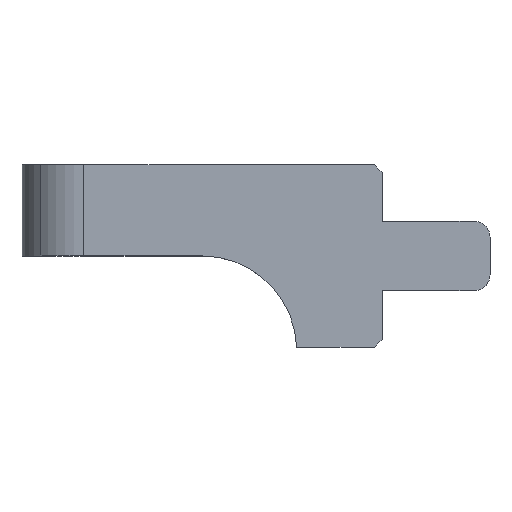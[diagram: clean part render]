
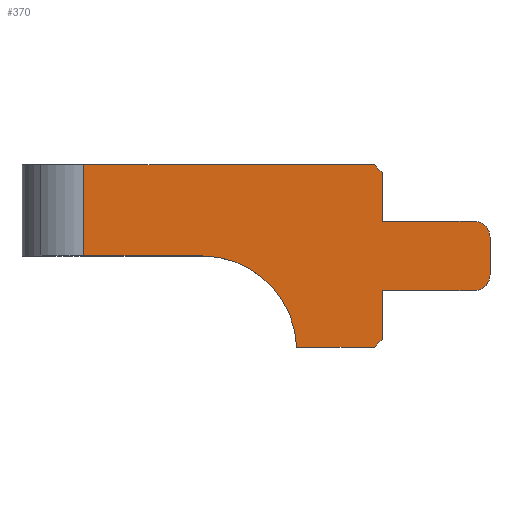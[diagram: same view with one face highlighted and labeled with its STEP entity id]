
A CAD part, top view. The second image highlights one B-rep face of the part: STEP entity #370.
In plain terms, the highlighted planar face has unit normal (0, 0, 1).
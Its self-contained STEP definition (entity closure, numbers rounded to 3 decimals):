
#4 = DIRECTION ( 'NONE',  ( -0.707, -0.707, 0. ) ) ;
#7 = CARTESIAN_POINT ( 'NONE',  ( 2.359, -3.087, 1.067 ) ) ;
#32 = DIRECTION ( 'NONE',  ( 0., 1., 0. ) ) ;
#40 = DIRECTION ( 'NONE',  ( 0., -1., 0. ) ) ;
#41 = LINE ( 'NONE', #339, #528 ) ;
#55 = CARTESIAN_POINT ( 'NONE',  ( 6.019, -0.811, 1.067 ) ) ;
#61 = CARTESIAN_POINT ( 'NONE',  ( -3.206, -0.207, 1.067 ) ) ;
#62 = VECTOR ( 'NONE', #478, 1000. ) ;
#65 = CIRCLE ( 'NONE', #229, 3.029 ) ;
#66 = VERTEX_POINT ( 'NONE', #672 ) ;
#72 = ORIENTED_EDGE ( 'NONE', *, *, #443, .F. ) ;
#75 = DIRECTION ( 'NONE',  ( 0., 1., 0. ) ) ;
#79 = VECTOR ( 'NONE', #32, 1000. ) ;
#80 = CARTESIAN_POINT ( 'NONE',  ( -6.995, 1.599, 1.067 ) ) ;
#91 = DIRECTION ( 'NONE',  ( 0., 0., 1. ) ) ;
#94 = ORIENTED_EDGE ( 'NONE', *, *, #477, .T. ) ;
#100 = CARTESIAN_POINT ( 'NONE',  ( 2.565, 0.904, 1.067 ) ) ;
#107 = ORIENTED_EDGE ( 'NONE', *, *, #491, .T. ) ;
#119 = ORIENTED_EDGE ( 'NONE', *, *, #495, .T. ) ;
#146 = VECTOR ( 'NONE', #75, 1000. ) ;
#156 = VERTEX_POINT ( 'NONE', #614 ) ;
#179 = CARTESIAN_POINT ( 'NONE',  ( 2.565, 2.466, 1.067 ) ) ;
#180 = VECTOR ( 'NONE', #442, 1000. ) ;
#181 = DIRECTION ( 'NONE',  ( 1., 0., 0. ) ) ;
#185 = DIRECTION ( 'NONE',  ( 0., 0., 1. ) ) ;
#199 = CARTESIAN_POINT ( 'NONE',  ( 2.565, -1.319, 1.067 ) ) ;
#202 = VECTOR ( 'NONE', #621, 1000. ) ;
#210 = CARTESIAN_POINT ( 'NONE',  ( -1.364, 0.479, 1.067 ) ) ;
#213 = VERTEX_POINT ( 'NONE', #456 ) ;
#219 = CARTESIAN_POINT ( 'NONE',  ( 5.511, -0.811, 1.067 ) ) ;
#229 = AXIS2_PLACEMENT_3D ( 'NONE', #696, #691, #343 ) ;
#234 = VECTOR ( 'NONE', #592, 1000. ) ;
#235 = AXIS2_PLACEMENT_3D ( 'NONE', #434, #91, #279 ) ;
#242 = AXIS2_PLACEMENT_3D ( 'NONE', #219, #658, #40 ) ;
#249 = CARTESIAN_POINT ( 'NONE',  ( 5.511, 0.904, 1.067 ) ) ;
#251 = PLANE ( 'NONE',  #274 ) ;
#252 = CARTESIAN_POINT ( 'NONE',  ( 2.565, 0.904, 1.067 ) ) ;
#254 = LINE ( 'NONE', #283, #412 ) ;
#258 = VERTEX_POINT ( 'NONE', #418 ) ;
#266 = ORIENTED_EDGE ( 'NONE', *, *, #479, .T. ) ;
#272 = CARTESIAN_POINT ( 'NONE',  ( 5.511, 0.904, 1.067 ) ) ;
#274 = AXIS2_PLACEMENT_3D ( 'NONE', #210, #185, #181 ) ;
#276 = DIRECTION ( 'NONE',  ( 1., 0., 0. ) ) ;
#277 = VECTOR ( 'NONE', #474, 1000. ) ;
#279 = DIRECTION ( 'NONE',  ( 1., 0., 0. ) ) ;
#283 = CARTESIAN_POINT ( 'NONE',  ( 2.565, -1.319, 1.067 ) ) ;
#313 = ORIENTED_EDGE ( 'NONE', *, *, #458, .T. ) ;
#339 = CARTESIAN_POINT ( 'NONE',  ( 2.016, 3.015, 1.067 ) ) ;
#343 = DIRECTION ( 'NONE',  ( -0.999, -0.034, 0. ) ) ;
#370 = ADVANCED_FACE ( 'NONE', ( #557 ), #251, .T. ) ;
#374 = LINE ( 'NONE', #475, #642 ) ;
#394 = LINE ( 'NONE', #272, #202 ) ;
#412 = VECTOR ( 'NONE', #703, 1000. ) ;
#418 = CARTESIAN_POINT ( 'NONE',  ( -0.178, -3.135, 1.067 ) ) ;
#422 = EDGE_CURVE ( 'NONE', #695, #468, #639, .T. ) ;
#428 = ORIENTED_EDGE ( 'NONE', *, *, #467, .T. ) ;
#434 = CARTESIAN_POINT ( 'NONE',  ( 5.511, 0.396, 1.067 ) ) ;
#442 = DIRECTION ( 'NONE',  ( -1., 0., 0. ) ) ;
#443 = EDGE_CURVE ( 'NONE', #66, #575, #618, .T. ) ;
#449 = ORIENTED_EDGE ( 'NONE', *, *, #484, .T. ) ;
#450 = CARTESIAN_POINT ( 'NONE',  ( -6.995, -0.207, 1.067 ) ) ;
#456 = CARTESIAN_POINT ( 'NONE',  ( 2.311, 2.72, 1.067 ) ) ;
#457 = LINE ( 'NONE', #601, #62 ) ;
#458 = EDGE_CURVE ( 'NONE', #258, #575, #598, .T. ) ;
#467 = EDGE_CURVE ( 'NONE', #66, #519, #587, .T. ) ;
#468 = VERTEX_POINT ( 'NONE', #547 ) ;
#470 = EDGE_CURVE ( 'NONE', #519, #156, #254, .T. ) ;
#471 = EDGE_CURVE ( 'NONE', #156, #577, #664, .T. ) ;
#474 = DIRECTION ( 'NONE',  ( 1., 0., 0. ) ) ;
#475 = CARTESIAN_POINT ( 'NONE',  ( -8.979, -0.207, 1.067 ) ) ;
#477 = EDGE_CURVE ( 'NONE', #577, #593, #457, .T. ) ;
#478 = DIRECTION ( 'NONE',  ( 0., 1., 0. ) ) ;
#479 = EDGE_CURVE ( 'NONE', #593, #602, #569, .T. ) ;
#484 = EDGE_CURVE ( 'NONE', #602, #623, #394, .T. ) ;
#487 = EDGE_CURVE ( 'NONE', #623, #681, #546, .T. ) ;
#490 = EDGE_CURVE ( 'NONE', #213, #681, #41, .T. ) ;
#491 = EDGE_CURVE ( 'NONE', #213, #468, #652, .T. ) ;
#493 = EDGE_CURVE ( 'NONE', #695, #670, #374, .T. ) ;
#495 = EDGE_CURVE ( 'NONE', #670, #258, #65, .T. ) ;
#507 = CARTESIAN_POINT ( 'NONE',  ( 6.019, 0.396, 1.067 ) ) ;
#519 = VERTEX_POINT ( 'NONE', #199 ) ;
#528 = VECTOR ( 'NONE', #631, 1000. ) ;
#533 = EDGE_LOOP ( 'NONE', ( #72, #428, #580, #675, #94, #266, #449, #596, #683, #107, #604, #697, #119, #313 ) ) ;
#546 = LINE ( 'NONE', #100, #234 ) ;
#547 = CARTESIAN_POINT ( 'NONE',  ( -6.995, 2.72, 1.067 ) ) ;
#557 = FACE_OUTER_BOUND ( 'NONE', #533, .T. ) ;
#569 = CIRCLE ( 'NONE', #235, 0.508 ) ;
#575 = VERTEX_POINT ( 'NONE', #638 ) ;
#577 = VERTEX_POINT ( 'NONE', #55 ) ;
#580 = ORIENTED_EDGE ( 'NONE', *, *, #470, .T. ) ;
#587 = LINE ( 'NONE', #690, #79 ) ;
#592 = DIRECTION ( 'NONE',  ( 0., 1., 0. ) ) ;
#593 = VERTEX_POINT ( 'NONE', #507 ) ;
#596 = ORIENTED_EDGE ( 'NONE', *, *, #487, .T. ) ;
#598 = LINE ( 'NONE', #619, #277 ) ;
#601 = CARTESIAN_POINT ( 'NONE',  ( 6.019, -0.811, 1.067 ) ) ;
#602 = VERTEX_POINT ( 'NONE', #249 ) ;
#604 = ORIENTED_EDGE ( 'NONE', *, *, #422, .F. ) ;
#614 = CARTESIAN_POINT ( 'NONE',  ( 5.511, -1.319, 1.067 ) ) ;
#618 = LINE ( 'NONE', #7, #702 ) ;
#619 = CARTESIAN_POINT ( 'NONE',  ( -0.178, -3.135, 1.067 ) ) ;
#621 = DIRECTION ( 'NONE',  ( -1., 0., 0. ) ) ;
#623 = VERTEX_POINT ( 'NONE', #252 ) ;
#631 = DIRECTION ( 'NONE',  ( 0.707, -0.707, 0. ) ) ;
#638 = CARTESIAN_POINT ( 'NONE',  ( 2.311, -3.135, 1.067 ) ) ;
#639 = LINE ( 'NONE', #80, #146 ) ;
#642 = VECTOR ( 'NONE', #276, 1000. ) ;
#652 = LINE ( 'NONE', #692, #180 ) ;
#658 = DIRECTION ( 'NONE',  ( 0., 0., 1. ) ) ;
#664 = CIRCLE ( 'NONE', #242, 0.508 ) ;
#670 = VERTEX_POINT ( 'NONE', #61 ) ;
#672 = CARTESIAN_POINT ( 'NONE',  ( 2.565, -2.881, 1.067 ) ) ;
#675 = ORIENTED_EDGE ( 'NONE', *, *, #471, .T. ) ;
#681 = VERTEX_POINT ( 'NONE', #179 ) ;
#683 = ORIENTED_EDGE ( 'NONE', *, *, #490, .F. ) ;
#690 = CARTESIAN_POINT ( 'NONE',  ( 2.565, -3.135, 1.067 ) ) ;
#691 = DIRECTION ( 'NONE',  ( 0., 0., -1. ) ) ;
#692 = CARTESIAN_POINT ( 'NONE',  ( 2.565, 2.72, 1.067 ) ) ;
#695 = VERTEX_POINT ( 'NONE', #450 ) ;
#696 = CARTESIAN_POINT ( 'NONE',  ( -3.206, -3.236, 1.067 ) ) ;
#697 = ORIENTED_EDGE ( 'NONE', *, *, #493, .T. ) ;
#702 = VECTOR ( 'NONE', #4, 1000. ) ;
#703 = DIRECTION ( 'NONE',  ( 1., 0., 0. ) ) ;
